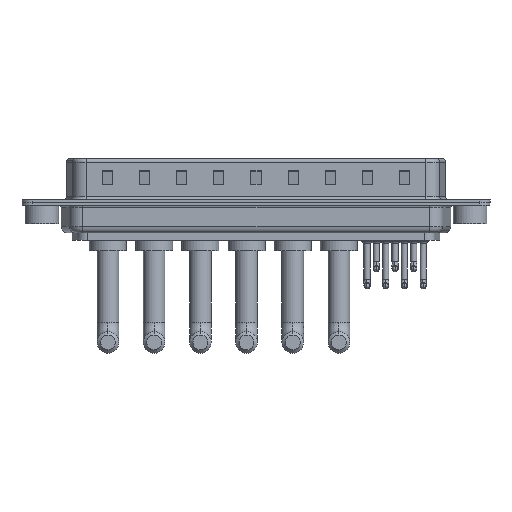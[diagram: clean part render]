
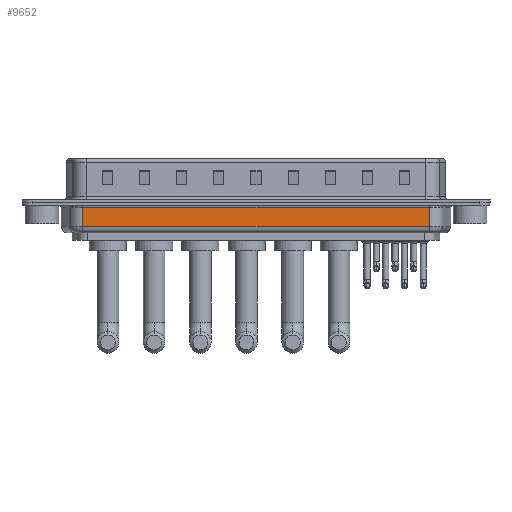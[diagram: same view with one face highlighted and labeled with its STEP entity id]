
A CAD part, front view. The second image highlights one B-rep face of the part: STEP entity #9652.
In plain terms, the highlighted planar face has unit normal (0, -1, 0).
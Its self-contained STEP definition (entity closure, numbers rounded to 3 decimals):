
#1143 = CARTESIAN_POINT ( 'NONE',  ( 57.469, -5.35, -3.5 ) ) ;
#1818 = CARTESIAN_POINT ( 'NONE',  ( 57.469, -5.35, -4.5 ) ) ;
#2006 = LINE ( 'NONE', #19007, #12041 ) ;
#2301 = VERTEX_POINT ( 'NONE', #1143 ) ;
#2946 = DIRECTION ( 'NONE',  ( 0., 0., 1. ) ) ;
#2988 = DIRECTION ( 'NONE',  ( 0., 1., 0. ) ) ;
#3321 = VECTOR ( 'NONE', #2946, 1000. ) ;
#3793 = LINE ( 'NONE', #1818, #23473 ) ;
#4444 = CARTESIAN_POINT ( 'NONE',  ( 6.031, -5.35, -3.5 ) ) ;
#5525 = ORIENTED_EDGE ( 'NONE', *, *, #20560, .T. ) ;
#6209 = CARTESIAN_POINT ( 'NONE',  ( 6.031, -5.35, -4.5 ) ) ;
#6717 = FACE_OUTER_BOUND ( 'NONE', #18270, .T. ) ;
#7338 = DIRECTION ( 'NONE',  ( -1., 0., 0. ) ) ;
#8578 = DIRECTION ( 'NONE',  ( -1., 0., 0. ) ) ;
#8693 = LINE ( 'NONE', #16279, #16800 ) ;
#9652 = ADVANCED_FACE ( 'NONE', ( #6717 ), #16040, .F. ) ;
#9673 = ORIENTED_EDGE ( 'NONE', *, *, #20902, .T. ) ;
#10102 = VERTEX_POINT ( 'NONE', #17614 ) ;
#10816 = EDGE_CURVE ( 'NONE', #11148, #18997, #19827, .T. ) ;
#11148 = VERTEX_POINT ( 'NONE', #4444 ) ;
#12041 = VECTOR ( 'NONE', #7338, 1000. ) ;
#12613 = ORIENTED_EDGE ( 'NONE', *, *, #18275, .T. ) ;
#12669 = ORIENTED_EDGE ( 'NONE', *, *, #10816, .F. ) ;
#13017 = DIRECTION ( 'NONE',  ( 0., 0., 1. ) ) ;
#14573 = CARTESIAN_POINT ( 'NONE',  ( 6.031, -5.35, -0.65 ) ) ;
#16040 = PLANE ( 'NONE',  #20705 ) ;
#16279 = CARTESIAN_POINT ( 'NONE',  ( 6.031, -5.35, -3.5 ) ) ;
#16800 = VECTOR ( 'NONE', #21962, 1000. ) ;
#17614 = CARTESIAN_POINT ( 'NONE',  ( 57.469, -5.35, -0.65 ) ) ;
#18270 = EDGE_LOOP ( 'NONE', ( #12669, #9673, #12613, #5525 ) ) ;
#18275 = EDGE_CURVE ( 'NONE', #2301, #10102, #3793, .T. ) ;
#18997 = VERTEX_POINT ( 'NONE', #14573 ) ;
#19007 = CARTESIAN_POINT ( 'NONE',  ( 6.031, -5.35, -0.65 ) ) ;
#19827 = LINE ( 'NONE', #21685, #3321 ) ;
#20560 = EDGE_CURVE ( 'NONE', #10102, #18997, #2006, .T. ) ;
#20705 = AXIS2_PLACEMENT_3D ( 'NONE', #6209, #2988, #8578 ) ;
#20902 = EDGE_CURVE ( 'NONE', #11148, #2301, #8693, .T. ) ;
#21685 = CARTESIAN_POINT ( 'NONE',  ( 6.031, -5.35, -4.5 ) ) ;
#21962 = DIRECTION ( 'NONE',  ( 1., 0., 0. ) ) ;
#23473 = VECTOR ( 'NONE', #13017, 1000. ) ;
